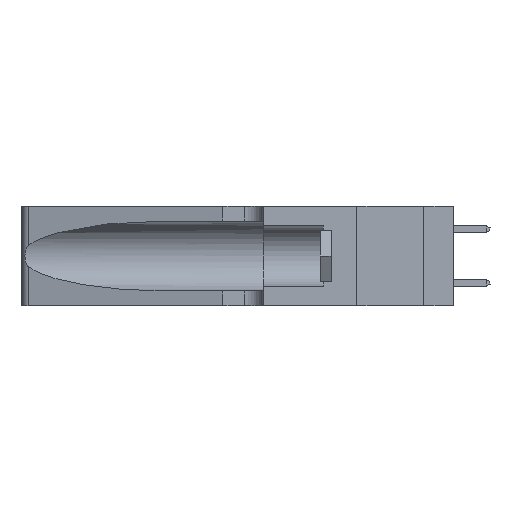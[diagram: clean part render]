
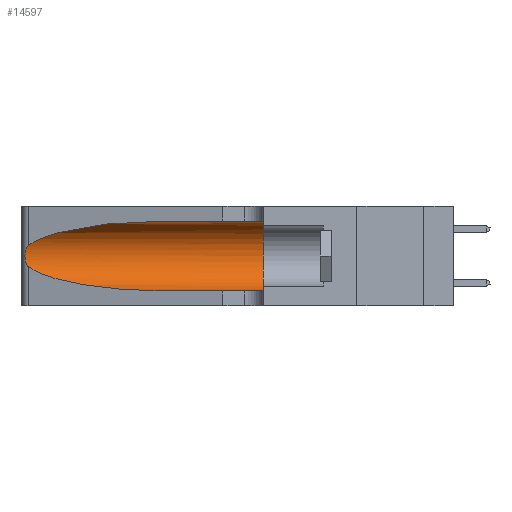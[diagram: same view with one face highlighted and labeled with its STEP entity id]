
A CAD part, left-side view. The second image highlights one B-rep face of the part: STEP entity #14597.
In plain terms, the highlighted cylindrical face has radius 3.308 mm (diameter 6.617 mm), a partial arc.
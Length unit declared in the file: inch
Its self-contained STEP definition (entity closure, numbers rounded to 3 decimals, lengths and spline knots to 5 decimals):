
#135 = ORIENTED_EDGE ( 'NONE', *, *, #16659, .T. ) ;
#639 = CARTESIAN_POINT ( 'NONE',  ( 0.2373, 1.15595, 0.28018 ) ) ;
#676 = CARTESIAN_POINT ( 'NONE',  ( 0.1305, 0.72297, 0.31525 ) ) ;
#995 = CARTESIAN_POINT ( 'NONE',  ( 0.26075, 1.23896, 0.19203 ) ) ;
#1053 = ORIENTED_EDGE ( 'NONE', *, *, #24789, .F. ) ;
#1098 = CARTESIAN_POINT ( 'NONE',  ( 0.25856, 1.23593, 0.16098 ) ) ;
#1123 = VERTEX_POINT ( 'NONE', #3314 ) ;
#1429 = EDGE_CURVE ( 'NONE', #5235, #6713, #25112, .T. ) ;
#2162 = ORIENTED_EDGE ( 'NONE', *, *, #28033, .T. ) ;
#3314 = CARTESIAN_POINT ( 'NONE',  ( 0.25487, 1.22718, 0.22369 ) ) ;
#3890 = DIRECTION ( 'NONE',  ( 0., 1., 0. ) ) ;
#4728 = CARTESIAN_POINT ( 'NONE',  ( 0.1305, 1.61858, 0.05475 ) ) ;
#5040 = AXIS2_PLACEMENT_3D ( 'NONE', #27896, #3890, #19102 ) ;
#5235 = VERTEX_POINT ( 'NONE', #8214 ) ;
#5427 = B_SPLINE_CURVE_WITH_KNOTS ( 'NONE', 3,
 ( #25905, #13168, #13619, #15826, #7248, #8977, #995, #22586, #9744, #1098, #9841, #13821, #18602, #20887 ),
 .UNSPECIFIED., .F., .F.,
 ( 4, 2, 2, 2, 2, 2, 4 ),
 ( 0., 0.00027, 0.00053, 0.00107, 0.0016, 0.00187, 0.00214 ),
 .UNSPECIFIED. ) ;
#5483 = LINE ( 'NONE', #23437, #27913 ) ;
#5671 = ORIENTED_EDGE ( 'NONE', *, *, #11090, .T. ) ;
#6529 = VERTEX_POINT ( 'NONE', #25683 ) ;
#6713 = VERTEX_POINT ( 'NONE', #7723 ) ;
#7066 = ORIENTED_EDGE ( 'NONE', *, *, #1429, .T. ) ;
#7248 = CARTESIAN_POINT ( 'NONE',  ( 0.25854, 1.2359, 0.20912 ) ) ;
#7487 = CARTESIAN_POINT ( 'NONE',  ( 0.18966, 0.96281, 0.31525 ) ) ;
#7723 = CARTESIAN_POINT ( 'NONE',  ( 0.1305, 0.72297, 0.05475 ) ) ;
#7754 = CARTESIAN_POINT ( 'NONE',  ( 0.25487, 1.22718, 0.14631 ) ) ;
#7799 = VECTOR ( 'NONE', #13376, 39.37008 ) ;
#8038 = CARTESIAN_POINT ( 'NONE',  ( 0.1305, 0.72297, 0.05475 ) ) ;
#8214 = CARTESIAN_POINT ( 'NONE',  ( 0.25487, 1.22718, 0.14631 ) ) ;
#8977 = CARTESIAN_POINT ( 'NONE',  ( 0.26018, 1.23835, 0.19895 ) ) ;
#9744 = CARTESIAN_POINT ( 'NONE',  ( 0.26017, 1.23833, 0.17102 ) ) ;
#9841 = CARTESIAN_POINT ( 'NONE',  ( 0.25789, 1.23486, 0.15765 ) ) ;
#10115 = CARTESIAN_POINT ( 'NONE',  ( 0.1305, 1.61858, 0.185 ) ) ;
#10134 = CARTESIAN_POINT ( 'NONE',  ( 0.18966, 0.96281, 0.05475 ) ) ;
#11090 = EDGE_CURVE ( 'NONE', #1123, #5235, #5427, .T. ) ;
#11224 = DIRECTION ( 'NONE',  ( 0., 0., -1. ) ) ;
#11293 = FACE_OUTER_BOUND ( 'NONE', #16766, .T. ) ;
#12282 = VERTEX_POINT ( 'NONE', #20615 ) ;
#12538 = EDGE_CURVE ( 'NONE', #6529, #12282, #19941, .T. ) ;
#13089 = AXIS2_PLACEMENT_3D ( 'NONE', #10115, #21453, #11224 ) ;
#13168 = CARTESIAN_POINT ( 'NONE',  ( 0.25555, 1.22994, 0.2215 ) ) ;
#13376 = DIRECTION ( 'NONE',  ( 0., -1., 0. ) ) ;
#13619 = CARTESIAN_POINT ( 'NONE',  ( 0.25639, 1.23184, 0.21858 ) ) ;
#13821 = CARTESIAN_POINT ( 'NONE',  ( 0.25639, 1.23186, 0.15144 ) ) ;
#14597 = ADVANCED_FACE ( 'NONE', ( #11293 ), #21180, .F. ) ;
#15337 = VERTEX_POINT ( 'NONE', #676 ) ;
#15826 = CARTESIAN_POINT ( 'NONE',  ( 0.25787, 1.23484, 0.2124 ) ) ;
#15870 = CARTESIAN_POINT ( 'NONE',  ( 0.25487, 1.22718, 0.22369 ) ) ;
#15968 = CARTESIAN_POINT ( 'NONE',  ( 0.1305, 0.72297, 0.31525 ) ) ;
#16659 = EDGE_CURVE ( 'NONE', #6713, #12282, #16863, .T. ) ;
#16766 = EDGE_LOOP ( 'NONE', ( #2162, #5671, #7066, #135, #17283, #1053 ) ) ;
#16863 = LINE ( 'NONE', #4728, #7799 ) ;
#17283 = ORIENTED_EDGE ( 'NONE', *, *, #12538, .F. ) ;
#18531 =( BOUNDED_CURVE ( )  B_SPLINE_CURVE ( 3, ( #15968, #7487, #639, #15870 ),
 .UNSPECIFIED., .F., .F. ) 
 B_SPLINE_CURVE_WITH_KNOTS ( ( 4, 4 ),
 ( 1.5708, 2.84003 ),
 .UNSPECIFIED. ) 
 CURVE ( )  GEOMETRIC_REPRESENTATION_ITEM ( )  RATIONAL_B_SPLINE_CURVE ( ( 1., 0.87, 0.87, 1. ) ) 
 REPRESENTATION_ITEM ( '' )  );
#18602 = CARTESIAN_POINT ( 'NONE',  ( 0.25555, 1.22993, 0.14849 ) ) ;
#18994 = CARTESIAN_POINT ( 'NONE',  ( 0.2373, 1.15595, 0.08982 ) ) ;
#19102 = DIRECTION ( 'NONE',  ( 0., 0., 1. ) ) ;
#19941 = CIRCLE ( 'NONE', #5040, 0.13025 ) ;
#20615 = CARTESIAN_POINT ( 'NONE',  ( 0.1305, 0.35, 0.05475 ) ) ;
#20887 = CARTESIAN_POINT ( 'NONE',  ( 0.25487, 1.22718, 0.14631 ) ) ;
#21180 = CYLINDRICAL_SURFACE ( 'NONE', #13089, 0.13025 ) ;
#21453 = DIRECTION ( 'NONE',  ( 0., -1., 0. ) ) ;
#22586 = CARTESIAN_POINT ( 'NONE',  ( 0.26075, 1.23896, 0.178 ) ) ;
#23437 = CARTESIAN_POINT ( 'NONE',  ( 0.1305, 1.61858, 0.31525 ) ) ;
#24789 = EDGE_CURVE ( 'NONE', #15337, #6529, #5483, .T. ) ;
#25112 =( BOUNDED_CURVE ( )  B_SPLINE_CURVE ( 3, ( #7754, #18994, #10134, #8038 ),
 .UNSPECIFIED., .F., .F. ) 
 B_SPLINE_CURVE_WITH_KNOTS ( ( 4, 4 ),
 ( 3.44316, 4.71239 ),
 .UNSPECIFIED. ) 
 CURVE ( )  GEOMETRIC_REPRESENTATION_ITEM ( )  RATIONAL_B_SPLINE_CURVE ( ( 1., 0.87, 0.87, 1. ) ) 
 REPRESENTATION_ITEM ( '' )  );
#25683 = CARTESIAN_POINT ( 'NONE',  ( 0.1305, 0.35, 0.31525 ) ) ;
#25905 = CARTESIAN_POINT ( 'NONE',  ( 0.25487, 1.22718, 0.22369 ) ) ;
#27791 = DIRECTION ( 'NONE',  ( 0., -1., 0. ) ) ;
#27896 = CARTESIAN_POINT ( 'NONE',  ( 0.1305, 0.35, 0.185 ) ) ;
#27913 = VECTOR ( 'NONE', #27791, 39.37008 ) ;
#28033 = EDGE_CURVE ( 'NONE', #15337, #1123, #18531, .T. ) ;
